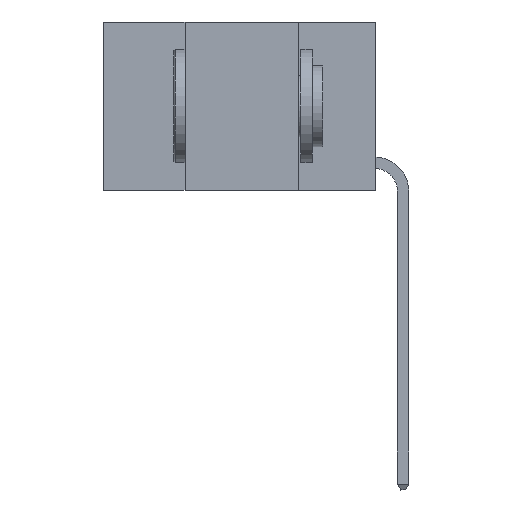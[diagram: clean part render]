
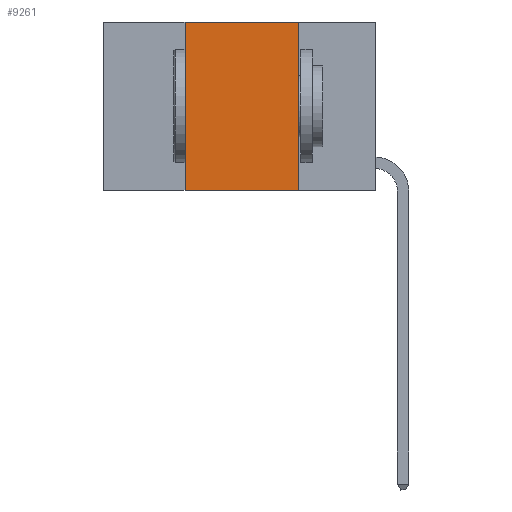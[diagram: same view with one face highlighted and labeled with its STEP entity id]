
A CAD part, left-side view. The second image highlights one B-rep face of the part: STEP entity #9261.
In plain terms, the highlighted planar face has unit normal (-1, 0, 0).
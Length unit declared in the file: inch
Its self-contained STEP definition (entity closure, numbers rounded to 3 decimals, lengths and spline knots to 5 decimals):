
#251 = AXIS2_PLACEMENT_3D ( 'NONE', #2023, #7004, #8179 ) ;
#770 = VECTOR ( 'NONE', #1133, 39.37008 ) ;
#826 = VERTEX_POINT ( 'NONE', #12863 ) ;
#883 = DIRECTION ( 'NONE',  ( 0., 0., 1. ) ) ;
#891 = EDGE_LOOP ( 'NONE', ( #2182, #7219, #3323, #10383 ) ) ;
#990 = LINE ( 'NONE', #10346, #770 ) ;
#1133 = DIRECTION ( 'NONE',  ( 0., 0., -1. ) ) ;
#2023 = CARTESIAN_POINT ( 'NONE',  ( 0., 0.6, 0. ) ) ;
#2182 = ORIENTED_EDGE ( 'NONE', *, *, #12203, .F. ) ;
#3323 = ORIENTED_EDGE ( 'NONE', *, *, #4928, .F. ) ;
#4021 = LINE ( 'NONE', #8151, #4911 ) ;
#4911 = VECTOR ( 'NONE', #12225, 39.37008 ) ;
#4928 = EDGE_CURVE ( 'NONE', #12509, #9440, #13241, .T. ) ;
#5033 = CARTESIAN_POINT ( 'NONE',  ( 0., 0.6, -0.37 ) ) ;
#5109 = FACE_OUTER_BOUND ( 'NONE', #891, .T. ) ;
#6246 = LINE ( 'NONE', #5033, #9202 ) ;
#7004 = DIRECTION ( 'NONE',  ( 1., 0., 0. ) ) ;
#7219 = ORIENTED_EDGE ( 'NONE', *, *, #11627, .F. ) ;
#8151 = CARTESIAN_POINT ( 'NONE',  ( 0., 0.6, 0. ) ) ;
#8179 = DIRECTION ( 'NONE',  ( 0., 0., -1. ) ) ;
#8234 = DIRECTION ( 'NONE',  ( 0., -1., 0. ) ) ;
#9202 = VECTOR ( 'NONE', #8234, 39.37008 ) ;
#9261 = ADVANCED_FACE ( 'NONE', ( #5109 ), #11182, .F. ) ;
#9300 = CARTESIAN_POINT ( 'NONE',  ( 0., 0.42, 0. ) ) ;
#9440 = VERTEX_POINT ( 'NONE', #12519 ) ;
#10346 = CARTESIAN_POINT ( 'NONE',  ( 0., 0.17, 0. ) ) ;
#10383 = ORIENTED_EDGE ( 'NONE', *, *, #13037, .T. ) ;
#11000 = VERTEX_POINT ( 'NONE', #11038 ) ;
#11038 = CARTESIAN_POINT ( 'NONE',  ( 0., 0.17, -0.37 ) ) ;
#11122 = CARTESIAN_POINT ( 'NONE',  ( 0., 0.42, -0.37 ) ) ;
#11182 = PLANE ( 'NONE',  #251 ) ;
#11627 = EDGE_CURVE ( 'NONE', #9440, #826, #4021, .T. ) ;
#12203 = EDGE_CURVE ( 'NONE', #826, #11000, #990, .T. ) ;
#12225 = DIRECTION ( 'NONE',  ( 0., -1., 0. ) ) ;
#12509 = VERTEX_POINT ( 'NONE', #11122 ) ;
#12519 = CARTESIAN_POINT ( 'NONE',  ( 0., 0.42, 0. ) ) ;
#12863 = CARTESIAN_POINT ( 'NONE',  ( 0., 0.17, 0. ) ) ;
#13037 = EDGE_CURVE ( 'NONE', #12509, #11000, #6246, .T. ) ;
#13241 = LINE ( 'NONE', #9300, #13259 ) ;
#13259 = VECTOR ( 'NONE', #883, 39.37008 ) ;
